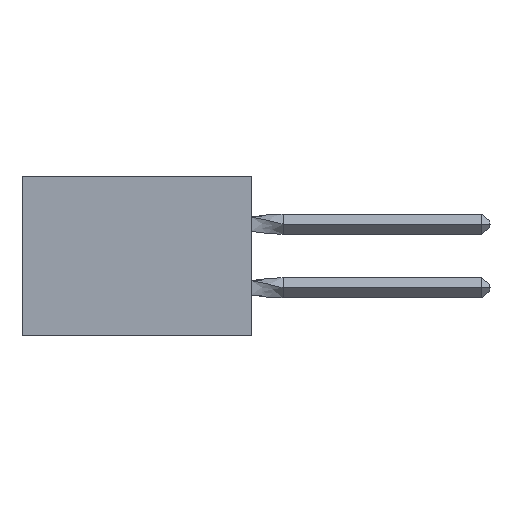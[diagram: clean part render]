
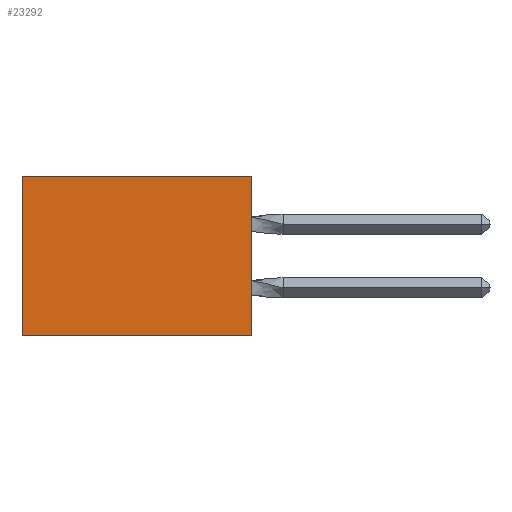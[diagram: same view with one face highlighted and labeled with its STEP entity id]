
A CAD part, left-side view. The second image highlights one B-rep face of the part: STEP entity #23292.
In plain terms, the highlighted planar face has unit normal (-1, 0, 0).
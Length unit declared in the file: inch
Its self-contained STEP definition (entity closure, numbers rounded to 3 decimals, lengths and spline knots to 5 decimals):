
#2695 = EDGE_LOOP ( 'NONE', ( #8914, #4155, #35803, #21528 ) ) ;
#4155 = ORIENTED_EDGE ( 'NONE', *, *, #4641, .F. ) ;
#4641 = EDGE_CURVE ( 'NONE', #17602, #33091, #11297, .T. ) ;
#6908 = CARTESIAN_POINT ( 'NONE',  ( 0.305, 0., 0. ) ) ;
#8164 = CARTESIAN_POINT ( 'NONE',  ( 0.305, 0.72, -0.5 ) ) ;
#8292 = DIRECTION ( 'NONE',  ( 0., 1., 0. ) ) ;
#8914 = ORIENTED_EDGE ( 'NONE', *, *, #19488, .T. ) ;
#10399 = CARTESIAN_POINT ( 'NONE',  ( 0.305, 0.72, 0. ) ) ;
#10639 = CARTESIAN_POINT ( 'NONE',  ( 0.305, 0., -0.5 ) ) ;
#10882 = DIRECTION ( 'NONE',  ( 1., 0., 0. ) ) ;
#11137 = DIRECTION ( 'NONE',  ( 0., 0., -1. ) ) ;
#11297 = LINE ( 'NONE', #11791, #19292 ) ;
#11332 = CARTESIAN_POINT ( 'NONE',  ( 0.305, 0.72, -0.5 ) ) ;
#11791 = CARTESIAN_POINT ( 'NONE',  ( 0.305, 0., -0.5 ) ) ;
#14845 = LINE ( 'NONE', #8164, #36598 ) ;
#15508 = DIRECTION ( 'NONE',  ( 0., 1., 0. ) ) ;
#16061 = VECTOR ( 'NONE', #31756, 39.37008 ) ;
#17602 = VERTEX_POINT ( 'NONE', #30892 ) ;
#18900 = EDGE_CURVE ( 'NONE', #21643, #22823, #20590, .T. ) ;
#19241 = PLANE ( 'NONE',  #28613 ) ;
#19292 = VECTOR ( 'NONE', #8292, 39.37008 ) ;
#19488 = EDGE_CURVE ( 'NONE', #22823, #33091, #14845, .T. ) ;
#20186 = CARTESIAN_POINT ( 'NONE',  ( 0.305, 0., -0.5 ) ) ;
#20590 = LINE ( 'NONE', #6908, #27667 ) ;
#20992 = EDGE_CURVE ( 'NONE', #21643, #17602, #32515, .T. ) ;
#21528 = ORIENTED_EDGE ( 'NONE', *, *, #18900, .T. ) ;
#21643 = VERTEX_POINT ( 'NONE', #32560 ) ;
#22823 = VERTEX_POINT ( 'NONE', #10399 ) ;
#23292 = ADVANCED_FACE ( 'NONE', ( #30569 ), #19241, .F. ) ;
#27667 = VECTOR ( 'NONE', #15508, 39.37008 ) ;
#28613 = AXIS2_PLACEMENT_3D ( 'NONE', #10639, #10882, #11137 ) ;
#30569 = FACE_OUTER_BOUND ( 'NONE', #2695, .T. ) ;
#30892 = CARTESIAN_POINT ( 'NONE',  ( 0.305, 0., -0.5 ) ) ;
#31110 = DIRECTION ( 'NONE',  ( 0., 0., -1. ) ) ;
#31756 = DIRECTION ( 'NONE',  ( 0., 0., -1. ) ) ;
#32515 = LINE ( 'NONE', #20186, #16061 ) ;
#32560 = CARTESIAN_POINT ( 'NONE',  ( 0.305, 0., 0. ) ) ;
#33091 = VERTEX_POINT ( 'NONE', #11332 ) ;
#35803 = ORIENTED_EDGE ( 'NONE', *, *, #20992, .F. ) ;
#36598 = VECTOR ( 'NONE', #31110, 39.37008 ) ;
